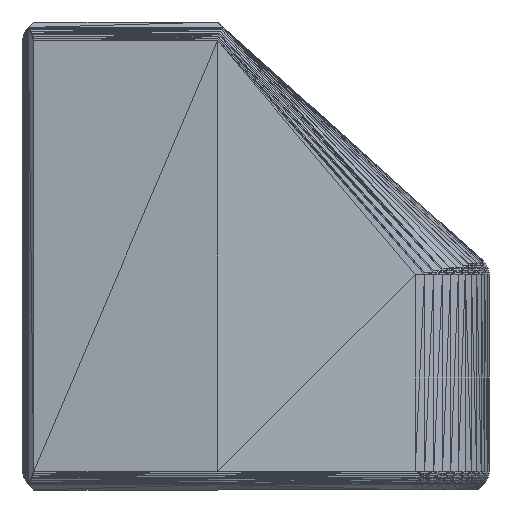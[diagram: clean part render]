
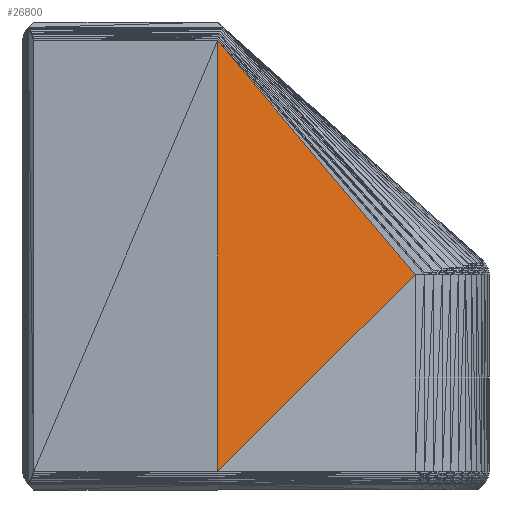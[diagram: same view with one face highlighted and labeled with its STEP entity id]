
A CAD part, front view. The second image highlights one B-rep face of the part: STEP entity #26800.
In plain terms, the highlighted planar face has unit normal (0.247, -0.969, 0).
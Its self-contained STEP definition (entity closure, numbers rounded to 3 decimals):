
#11288 = VERTEX_POINT('',#11289);
#11289 = CARTESIAN_POINT('',(26.655,-19.24,
    -122.748));
#11303 = PLANE('',#11304);
#11304 = AXIS2_PLACEMENT_3D('',#11305,#11306,#11307);
#11305 = CARTESIAN_POINT('',(43.9,-14.851,
    -113.387));
#11306 = DIRECTION('',(0.247,-0.969,0.
    ));
#11307 = DIRECTION('',(-0.969,-0.247,0.));
#17712 = VERTEX_POINT('',#17713);
#17713 = CARTESIAN_POINT('',(26.655,-19.24,
    -64.328));
#17757 = PLANE('',#17758);
#17758 = AXIS2_PLACEMENT_3D('',#17759,#17760,#17761);
#17759 = CARTESIAN_POINT('',(40.583,-15.691,
    -80.447));
#17760 = DIRECTION('',(0.259,-0.966,0.011
    ));
#17761 = DIRECTION('',(-0.966,-0.259,0.));
#17797 = EDGE_CURVE('',#17712,#17798,#17800,.T.);
#17798 = VERTEX_POINT('',#17799);
#17799 = CARTESIAN_POINT('',(53.44,-12.422,
    -96.077));
#17800 = SURFACE_CURVE('',#17801,(#17805,#17812),.PCURVE_S1.);
#17801 = LINE('',#17802,#17803);
#17802 = CARTESIAN_POINT('',(26.655,-19.24,
    -64.328));
#17803 = VECTOR('',#17804,1.);
#17804 = DIRECTION('',(0.636,0.162,-0.754));
#17805 = PCURVE('',#17757,#17806);
#17806 = DEFINITIONAL_REPRESENTATION('',(#17807),#17811);
#17807 = LINE('',#17808,#17809);
#17808 = CARTESIAN_POINT('',(14.372,-16.119));
#17809 = VECTOR('',#17810,1.);
#17810 = DIRECTION('',(-0.657,0.754));
#17811 = ( GEOMETRIC_REPRESENTATION_CONTEXT(2) 
PARAMETRIC_REPRESENTATION_CONTEXT() REPRESENTATION_CONTEXT('2D SPACE',''
  ) );
#17812 = PCURVE('',#17813,#17818);
#17813 = PLANE('',#17814);
#17814 = AXIS2_PLACEMENT_3D('',#17815,#17816,#17817);
#17815 = CARTESIAN_POINT('',(34.416,-17.265,
    -93.886));
#17816 = DIRECTION('',(0.247,-0.969,
    0.));
#17817 = DIRECTION('',(-0.969,-0.247,
    0.));
#17818 = DEFINITIONAL_REPRESENTATION('',(#17819),#17822);
#17819 = B_SPLINE_CURVE_WITH_KNOTS('',1,(#17820,#17821),.UNSPECIFIED.,
  .F.,.F.,(2,2),(0.,42.094),.PIECEWISE_BEZIER_KNOTS.);
#17820 = CARTESIAN_POINT('',(8.008,-29.558));
#17821 = CARTESIAN_POINT('',(-19.631,2.19));
#17822 = ( GEOMETRIC_REPRESENTATION_CONTEXT(2) 
PARAMETRIC_REPRESENTATION_CONTEXT() REPRESENTATION_CONTEXT('2D SPACE',''
  ) );
#17957 = PLANE('',#17958);
#17958 = AXIS2_PLACEMENT_3D('',#17959,#17960,#17961);
#17959 = CARTESIAN_POINT('',(19.137,-19.24,
    -98.502));
#17960 = DIRECTION('',(-0.,-1.,-0.));
#17961 = DIRECTION('',(0.,0.,-1.));
#17972 = EDGE_CURVE('',#11288,#17712,#17973,.T.);
#17973 = SURFACE_CURVE('',#17974,(#17978,#17985),.PCURVE_S1.);
#17974 = LINE('',#17975,#17976);
#17975 = CARTESIAN_POINT('',(26.655,-19.24,
    -122.748));
#17976 = VECTOR('',#17977,1.);
#17977 = DIRECTION('',(0.,0.,1.));
#17978 = PCURVE('',#17957,#17979);
#17979 = DEFINITIONAL_REPRESENTATION('',(#17980),#17984);
#17980 = LINE('',#17981,#17982);
#17981 = CARTESIAN_POINT('',(24.246,7.519));
#17982 = VECTOR('',#17983,1.);
#17983 = DIRECTION('',(-1.,0.));
#17984 = ( GEOMETRIC_REPRESENTATION_CONTEXT(2) 
PARAMETRIC_REPRESENTATION_CONTEXT() REPRESENTATION_CONTEXT('2D SPACE',''
  ) );
#17985 = PCURVE('',#17813,#17986);
#17986 = DEFINITIONAL_REPRESENTATION('',(#17987),#17990);
#17987 = B_SPLINE_CURVE_WITH_KNOTS('',1,(#17988,#17989),.UNSPECIFIED.,
  .F.,.F.,(2,2),(0.,58.42),.PIECEWISE_BEZIER_KNOTS.);
#17988 = CARTESIAN_POINT('',(8.008,28.862));
#17989 = CARTESIAN_POINT('',(8.008,-29.558));
#17990 = ( GEOMETRIC_REPRESENTATION_CONTEXT(2) 
PARAMETRIC_REPRESENTATION_CONTEXT() REPRESENTATION_CONTEXT('2D SPACE',''
  ) );
#26800 = ADVANCED_FACE('',(#26801),#17813,.T.);
#26801 = FACE_BOUND('',#26802,.T.);
#26802 = EDGE_LOOP('',(#26803,#26804,#26824));
#26803 = ORIENTED_EDGE('',*,*,#17972,.F.);
#26804 = ORIENTED_EDGE('',*,*,#26805,.T.);
#26805 = EDGE_CURVE('',#11288,#17798,#26806,.T.);
#26806 = SURFACE_CURVE('',#26807,(#26811,#26818),.PCURVE_S1.);
#26807 = LINE('',#26808,#26809);
#26808 = CARTESIAN_POINT('',(26.655,-19.24,
    -122.748));
#26809 = VECTOR('',#26810,1.);
#26810 = DIRECTION('',(0.697,0.178,0.694));
#26811 = PCURVE('',#17813,#26812);
#26812 = DEFINITIONAL_REPRESENTATION('',(#26813),#26817);
#26813 = LINE('',#26814,#26815);
#26814 = CARTESIAN_POINT('',(8.008,28.862));
#26815 = VECTOR('',#26816,1.);
#26816 = DIRECTION('',(-0.72,-0.694));
#26817 = ( GEOMETRIC_REPRESENTATION_CONTEXT(2) 
PARAMETRIC_REPRESENTATION_CONTEXT() REPRESENTATION_CONTEXT('2D SPACE',''
  ) );
#26818 = PCURVE('',#11303,#26819);
#26819 = DEFINITIONAL_REPRESENTATION('',(#26820),#26823);
#26820 = B_SPLINE_CURVE_WITH_KNOTS('',1,(#26821,#26822),.UNSPECIFIED.,
  .F.,.F.,(2,2),(0.,38.409),.PIECEWISE_BEZIER_KNOTS.);
#26821 = CARTESIAN_POINT('',(17.795,9.361));
#26822 = CARTESIAN_POINT('',(-9.845,-17.31));
#26823 = ( GEOMETRIC_REPRESENTATION_CONTEXT(2) 
PARAMETRIC_REPRESENTATION_CONTEXT() REPRESENTATION_CONTEXT('2D SPACE',''
  ) );
#26824 = ORIENTED_EDGE('',*,*,#17797,.F.);
